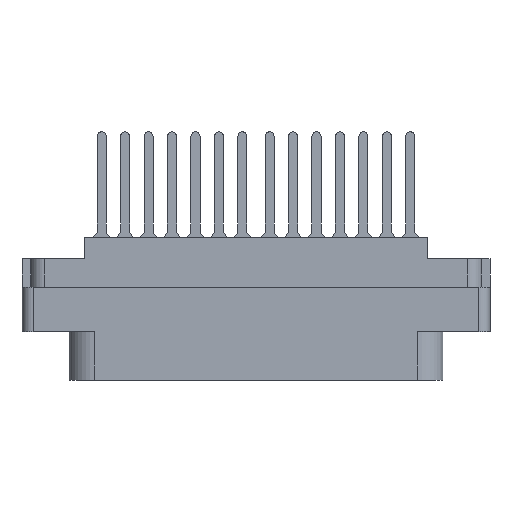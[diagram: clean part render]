
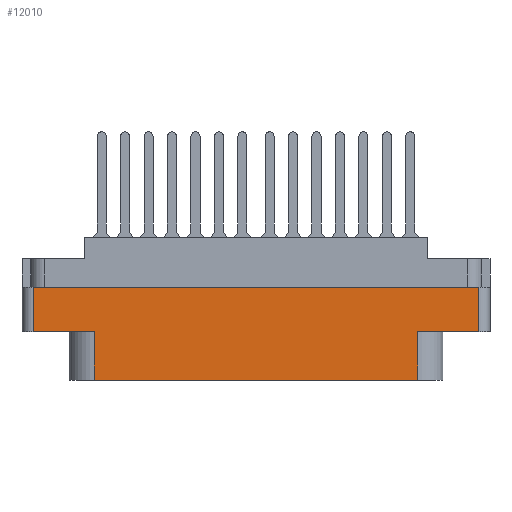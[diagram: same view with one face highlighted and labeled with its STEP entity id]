
A CAD part, front view. The second image highlights one B-rep face of the part: STEP entity #12010.
In plain terms, the highlighted planar face has unit normal (0, -1, 0).
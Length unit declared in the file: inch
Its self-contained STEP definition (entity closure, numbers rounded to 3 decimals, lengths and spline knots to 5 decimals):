
#335 = CARTESIAN_POINT ( 'NONE',  ( 0., -0.438, -0.52 ) ) ;
#995 = ORIENTED_EDGE ( 'NONE', *, *, #25782, .T. ) ;
#1263 = VECTOR ( 'NONE', #30299, 39.37008 ) ;
#2455 = VERTEX_POINT ( 'NONE', #8987 ) ;
#2586 = VECTOR ( 'NONE', #7844, 39.37008 ) ;
#4460 = AXIS2_PLACEMENT_3D ( 'NONE', #30014, #7226, #33720 ) ;
#5789 = ORIENTED_EDGE ( 'NONE', *, *, #24854, .F. ) ;
#5812 = CARTESIAN_POINT ( 'NONE',  ( -0.895, -0.438, -0.52 ) ) ;
#6605 = EDGE_CURVE ( 'NONE', #48617, #31111, #38658, .T. ) ;
#7226 = DIRECTION ( 'NONE',  ( 0., -1., 0. ) ) ;
#7334 = DIRECTION ( 'NONE',  ( 0., 0., -1. ) ) ;
#7662 = LINE ( 'NONE', #14636, #13661 ) ;
#7844 = DIRECTION ( 'NONE',  ( 0., 0., 1. ) ) ;
#8555 = ORIENTED_EDGE ( 'NONE', *, *, #39929, .T. ) ;
#8987 = CARTESIAN_POINT ( 'NONE',  ( 0.895, -0.438, -0.789 ) ) ;
#12010 = ADVANCED_FACE ( 'NONE', ( #44068 ), #49365, .T. ) ;
#12268 = VERTEX_POINT ( 'NONE', #31846 ) ;
#13075 = ORIENTED_EDGE ( 'NONE', *, *, #41182, .F. ) ;
#13657 = CARTESIAN_POINT ( 'NONE',  ( -0.895, -0.438, -0.789 ) ) ;
#13661 = VECTOR ( 'NONE', #37963, 39.37008 ) ;
#14636 = CARTESIAN_POINT ( 'NONE',  ( 1.2335, -0.438, -0.789 ) ) ;
#15321 = CARTESIAN_POINT ( 'NONE',  ( 0., -0.438, -0.274 ) ) ;
#16139 = CARTESIAN_POINT ( 'NONE',  ( 0.895, -0.438, -0.52 ) ) ;
#18379 = EDGE_CURVE ( 'NONE', #12268, #19529, #7662, .T. ) ;
#19529 = VERTEX_POINT ( 'NONE', #23344 ) ;
#21821 = DIRECTION ( 'NONE',  ( 1., 0., 0. ) ) ;
#23344 = CARTESIAN_POINT ( 'NONE',  ( 1.2335, -0.438, -0.274 ) ) ;
#23511 = DIRECTION ( 'NONE',  ( -1., 0., 0. ) ) ;
#24757 = DIRECTION ( 'NONE',  ( 0., 0., -1. ) ) ;
#24854 = EDGE_CURVE ( 'NONE', #12268, #25429, #28132, .T. ) ;
#25297 = EDGE_LOOP ( 'NONE', ( #46831, #30210, #13075, #8555, #995, #29340, #5789, #49174 ) ) ;
#25429 = VERTEX_POINT ( 'NONE', #16139 ) ;
#25603 = CARTESIAN_POINT ( 'NONE',  ( 0., -0.438, -0.52 ) ) ;
#25782 = EDGE_CURVE ( 'NONE', #34747, #2455, #26804, .T. ) ;
#26804 = LINE ( 'NONE', #47973, #44781 ) ;
#28132 = LINE ( 'NONE', #335, #37217 ) ;
#28135 = VERTEX_POINT ( 'NONE', #5812 ) ;
#29335 = CARTESIAN_POINT ( 'NONE',  ( -1.2335, -0.438, -0.789 ) ) ;
#29340 = ORIENTED_EDGE ( 'NONE', *, *, #31951, .T. ) ;
#30014 = CARTESIAN_POINT ( 'NONE',  ( -1.2955, -0.438, -0.789 ) ) ;
#30210 = ORIENTED_EDGE ( 'NONE', *, *, #6605, .T. ) ;
#30299 = DIRECTION ( 'NONE',  ( 1., 0., 0. ) ) ;
#30338 = CARTESIAN_POINT ( 'NONE',  ( 0.895, -0.438, -0.52 ) ) ;
#31111 = VERTEX_POINT ( 'NONE', #49344 ) ;
#31846 = CARTESIAN_POINT ( 'NONE',  ( 1.2335, -0.438, -0.52 ) ) ;
#31951 = EDGE_CURVE ( 'NONE', #2455, #25429, #40363, .T. ) ;
#33720 = DIRECTION ( 'NONE',  ( 0., 0., -1. ) ) ;
#33876 = VECTOR ( 'NONE', #24757, 39.37008 ) ;
#34747 = VERTEX_POINT ( 'NONE', #13657 ) ;
#35378 = LINE ( 'NONE', #25603, #44260 ) ;
#37217 = VECTOR ( 'NONE', #23511, 39.37008 ) ;
#37841 = CARTESIAN_POINT ( 'NONE',  ( -0.895, -0.438, -0.789 ) ) ;
#37963 = DIRECTION ( 'NONE',  ( 0., 0., 1. ) ) ;
#38658 = LINE ( 'NONE', #29335, #33876 ) ;
#39929 = EDGE_CURVE ( 'NONE', #28135, #34747, #41117, .T. ) ;
#40363 = LINE ( 'NONE', #30338, #2586 ) ;
#41117 = LINE ( 'NONE', #37841, #42300 ) ;
#41182 = EDGE_CURVE ( 'NONE', #28135, #31111, #35378, .T. ) ;
#42300 = VECTOR ( 'NONE', #7334, 39.37008 ) ;
#42922 = CARTESIAN_POINT ( 'NONE',  ( -1.2335, -0.438, -0.274 ) ) ;
#43607 = EDGE_CURVE ( 'NONE', #48617, #19529, #48519, .T. ) ;
#44068 = FACE_OUTER_BOUND ( 'NONE', #25297, .T. ) ;
#44260 = VECTOR ( 'NONE', #44682, 39.37008 ) ;
#44682 = DIRECTION ( 'NONE',  ( -1., 0., 0. ) ) ;
#44781 = VECTOR ( 'NONE', #21821, 39.37008 ) ;
#46831 = ORIENTED_EDGE ( 'NONE', *, *, #43607, .F. ) ;
#47973 = CARTESIAN_POINT ( 'NONE',  ( -1.2955, -0.438, -0.789 ) ) ;
#48519 = LINE ( 'NONE', #15321, #1263 ) ;
#48617 = VERTEX_POINT ( 'NONE', #42922 ) ;
#49174 = ORIENTED_EDGE ( 'NONE', *, *, #18379, .T. ) ;
#49344 = CARTESIAN_POINT ( 'NONE',  ( -1.2335, -0.438, -0.52 ) ) ;
#49365 = PLANE ( 'NONE',  #4460 ) ;
